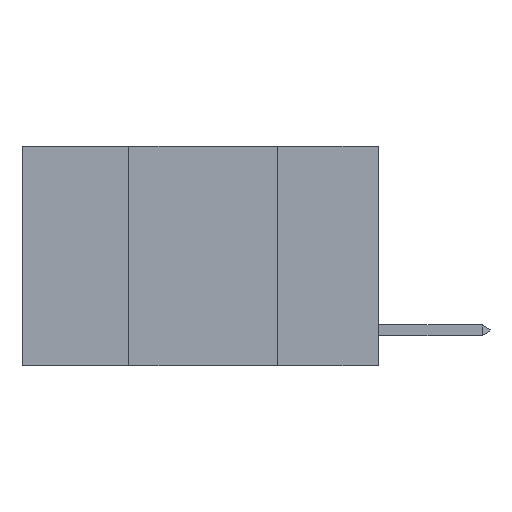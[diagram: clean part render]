
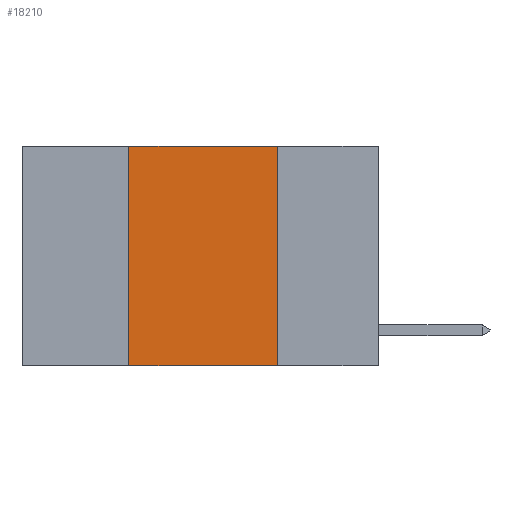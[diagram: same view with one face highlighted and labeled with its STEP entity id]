
A CAD part, left-side view. The second image highlights one B-rep face of the part: STEP entity #18210.
In plain terms, the highlighted planar face has unit normal (-1, 0, 0).
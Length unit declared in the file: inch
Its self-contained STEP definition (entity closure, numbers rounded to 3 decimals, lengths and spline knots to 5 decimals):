
#769 = CARTESIAN_POINT ( 'NONE',  ( 0., 0.42, 0. ) ) ;
#1365 = DIRECTION ( 'NONE',  ( 0., -1., 0. ) ) ;
#1440 = DIRECTION ( 'NONE',  ( 0., 0., -1. ) ) ;
#2715 = ORIENTED_EDGE ( 'NONE', *, *, #15439, .F. ) ;
#2744 = CARTESIAN_POINT ( 'NONE',  ( 0., 0.6, -0.37 ) ) ;
#2890 = EDGE_LOOP ( 'NONE', ( #14401, #8967, #2715, #12167 ) ) ;
#3353 = CARTESIAN_POINT ( 'NONE',  ( 0., 0.42, 0. ) ) ;
#3789 = FACE_OUTER_BOUND ( 'NONE', #2890, .T. ) ;
#3848 = LINE ( 'NONE', #2744, #12424 ) ;
#4010 = VECTOR ( 'NONE', #9826, 39.37008 ) ;
#4723 = LINE ( 'NONE', #16712, #11952 ) ;
#5437 = CARTESIAN_POINT ( 'NONE',  ( 0., 0.42, -0.37 ) ) ;
#5677 = PLANE ( 'NONE',  #11678 ) ;
#6385 = VERTEX_POINT ( 'NONE', #5437 ) ;
#6668 = DIRECTION ( 'NONE',  ( 0., 0., -1. ) ) ;
#7248 = VERTEX_POINT ( 'NONE', #15954 ) ;
#7590 = EDGE_CURVE ( 'NONE', #9898, #7248, #11656, .T. ) ;
#8085 = CARTESIAN_POINT ( 'NONE',  ( 0., 0.17, -0.37 ) ) ;
#8371 = CARTESIAN_POINT ( 'NONE',  ( 0., 0.6, 0. ) ) ;
#8967 = ORIENTED_EDGE ( 'NONE', *, *, #7590, .F. ) ;
#9826 = DIRECTION ( 'NONE',  ( 0., -1., 0. ) ) ;
#9898 = VERTEX_POINT ( 'NONE', #3353 ) ;
#10049 = DIRECTION ( 'NONE',  ( 1., 0., 0. ) ) ;
#10098 = VERTEX_POINT ( 'NONE', #8085 ) ;
#11656 = LINE ( 'NONE', #8371, #4010 ) ;
#11678 = AXIS2_PLACEMENT_3D ( 'NONE', #17115, #10049, #1440 ) ;
#11952 = VECTOR ( 'NONE', #6668, 39.37008 ) ;
#12167 = ORIENTED_EDGE ( 'NONE', *, *, #14487, .T. ) ;
#12424 = VECTOR ( 'NONE', #1365, 39.37008 ) ;
#14063 = VECTOR ( 'NONE', #17933, 39.37008 ) ;
#14401 = ORIENTED_EDGE ( 'NONE', *, *, #17302, .F. ) ;
#14487 = EDGE_CURVE ( 'NONE', #6385, #10098, #3848, .T. ) ;
#15439 = EDGE_CURVE ( 'NONE', #6385, #9898, #17793, .T. ) ;
#15954 = CARTESIAN_POINT ( 'NONE',  ( 0., 0.17, 0. ) ) ;
#16712 = CARTESIAN_POINT ( 'NONE',  ( 0., 0.17, 0. ) ) ;
#17115 = CARTESIAN_POINT ( 'NONE',  ( 0., 0.6, 0. ) ) ;
#17302 = EDGE_CURVE ( 'NONE', #7248, #10098, #4723, .T. ) ;
#17793 = LINE ( 'NONE', #769, #14063 ) ;
#17933 = DIRECTION ( 'NONE',  ( 0., 0., 1. ) ) ;
#18210 = ADVANCED_FACE ( 'NONE', ( #3789 ), #5677, .F. ) ;
